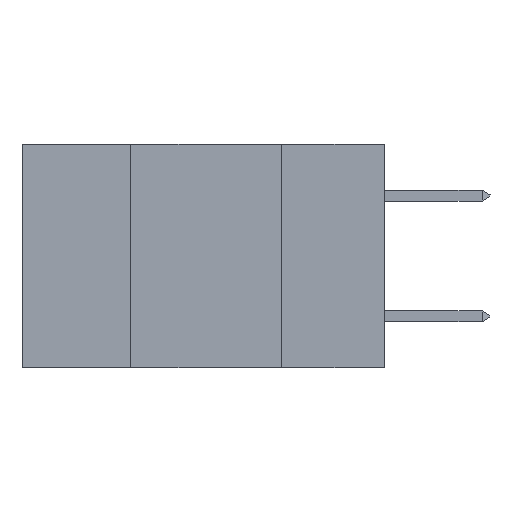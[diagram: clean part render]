
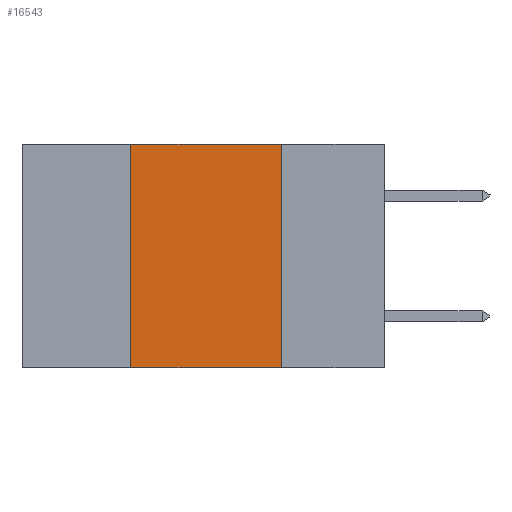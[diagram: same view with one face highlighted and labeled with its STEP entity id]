
A CAD part, left-side view. The second image highlights one B-rep face of the part: STEP entity #16543.
In plain terms, the highlighted planar face has unit normal (-1, 0, 0).
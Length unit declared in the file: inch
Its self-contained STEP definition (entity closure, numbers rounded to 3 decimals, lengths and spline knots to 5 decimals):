
#2051 = EDGE_LOOP ( 'NONE', ( #14745, #17104, #14505, #10281 ) ) ;
#3600 = CARTESIAN_POINT ( 'NONE',  ( 0., 0.17, 0. ) ) ;
#3628 = DIRECTION ( 'NONE',  ( 1., 0., 0. ) ) ;
#4451 = CARTESIAN_POINT ( 'NONE',  ( 0., 0.6, 0. ) ) ;
#5575 = LINE ( 'NONE', #4451, #7591 ) ;
#6817 = EDGE_CURVE ( 'NONE', #6952, #29218, #34258, .T. ) ;
#6884 = DIRECTION ( 'NONE',  ( 0., 0., -1. ) ) ;
#6952 = VERTEX_POINT ( 'NONE', #41078 ) ;
#7348 = LINE ( 'NONE', #3600, #9401 ) ;
#7591 = VECTOR ( 'NONE', #30558, 39.37008 ) ;
#8458 = CARTESIAN_POINT ( 'NONE',  ( 0., 0.17, -0.37 ) ) ;
#8864 = DIRECTION ( 'NONE',  ( 0., -1., 0. ) ) ;
#9401 = VECTOR ( 'NONE', #16207, 39.37008 ) ;
#10281 = ORIENTED_EDGE ( 'NONE', *, *, #6817, .T. ) ;
#14505 = ORIENTED_EDGE ( 'NONE', *, *, #23984, .F. ) ;
#14745 = ORIENTED_EDGE ( 'NONE', *, *, #33543, .F. ) ;
#15197 = FACE_OUTER_BOUND ( 'NONE', #2051, .T. ) ;
#15656 = VERTEX_POINT ( 'NONE', #16636 ) ;
#16207 = DIRECTION ( 'NONE',  ( 0., 0., -1. ) ) ;
#16507 = PLANE ( 'NONE',  #33096 ) ;
#16543 = ADVANCED_FACE ( 'NONE', ( #15197 ), #16507, .F. ) ;
#16636 = CARTESIAN_POINT ( 'NONE',  ( 0., 0.17, 0. ) ) ;
#17104 = ORIENTED_EDGE ( 'NONE', *, *, #26395, .F. ) ;
#19700 = CARTESIAN_POINT ( 'NONE',  ( 0., 0.6, 0. ) ) ;
#23938 = LINE ( 'NONE', #24692, #37031 ) ;
#23984 = EDGE_CURVE ( 'NONE', #6952, #35860, #23938, .T. ) ;
#24692 = CARTESIAN_POINT ( 'NONE',  ( 0., 0.42, 0. ) ) ;
#25375 = CARTESIAN_POINT ( 'NONE',  ( 0., 0.42, 0. ) ) ;
#26395 = EDGE_CURVE ( 'NONE', #35860, #15656, #5575, .T. ) ;
#27978 = DIRECTION ( 'NONE',  ( 0., 0., 1. ) ) ;
#29218 = VERTEX_POINT ( 'NONE', #8458 ) ;
#30558 = DIRECTION ( 'NONE',  ( 0., -1., 0. ) ) ;
#33096 = AXIS2_PLACEMENT_3D ( 'NONE', #19700, #3628, #6884 ) ;
#33543 = EDGE_CURVE ( 'NONE', #15656, #29218, #7348, .T. ) ;
#33781 = VECTOR ( 'NONE', #8864, 39.37008 ) ;
#34258 = LINE ( 'NONE', #34327, #33781 ) ;
#34327 = CARTESIAN_POINT ( 'NONE',  ( 0., 0.6, -0.37 ) ) ;
#35860 = VERTEX_POINT ( 'NONE', #25375 ) ;
#37031 = VECTOR ( 'NONE', #27978, 39.37008 ) ;
#41078 = CARTESIAN_POINT ( 'NONE',  ( 0., 0.42, -0.37 ) ) ;
